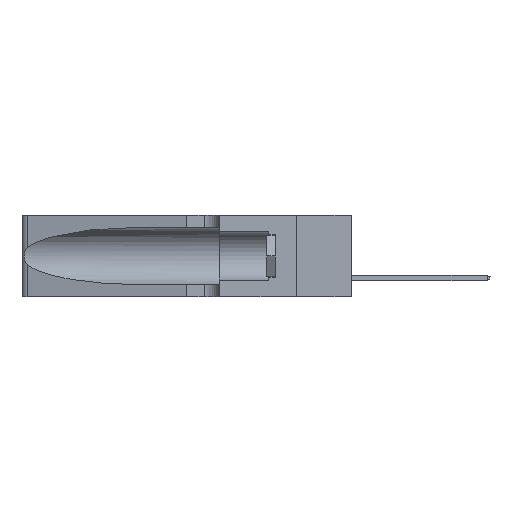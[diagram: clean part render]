
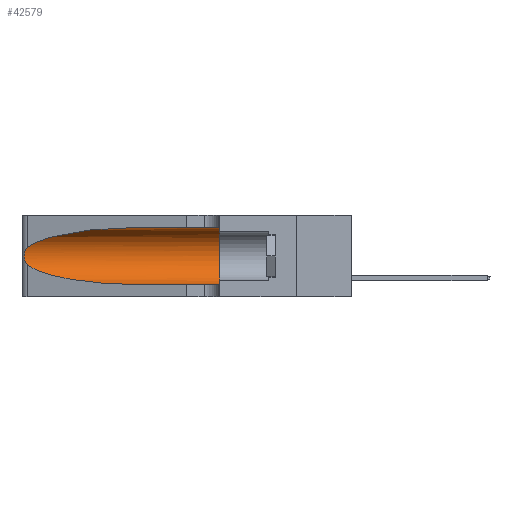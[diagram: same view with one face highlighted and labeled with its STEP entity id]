
A CAD part, left-side view. The second image highlights one B-rep face of the part: STEP entity #42579.
In plain terms, the highlighted cylindrical face has radius 3.308 mm (diameter 6.617 mm), a partial arc.
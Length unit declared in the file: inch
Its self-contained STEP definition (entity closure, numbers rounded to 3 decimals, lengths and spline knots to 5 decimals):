
#1730 = EDGE_LOOP ( 'NONE', ( #22844, #33410, #13693, #36216, #8523, #17052 ) ) ;
#2584 = DIRECTION ( 'NONE',  ( 0., -1., 0. ) ) ;
#3166 = CARTESIAN_POINT ( 'NONE',  ( 0.26075, 1.23896, 0.19203 ) ) ;
#6509 = VERTEX_POINT ( 'NONE', #18634 ) ;
#6924 = CARTESIAN_POINT ( 'NONE',  ( 0.1305, 1.61858, 0.05475 ) ) ;
#7042 = CARTESIAN_POINT ( 'NONE',  ( 0.25856, 1.23593, 0.16098 ) ) ;
#7304 = EDGE_CURVE ( 'NONE', #24124, #16155, #22294, .T. ) ;
#7346 = CARTESIAN_POINT ( 'NONE',  ( 0.25555, 1.22993, 0.14849 ) ) ;
#7727 = VERTEX_POINT ( 'NONE', #22287 ) ;
#8378 = DIRECTION ( 'NONE',  ( 0., 1., 0. ) ) ;
#8523 = ORIENTED_EDGE ( 'NONE', *, *, #11274, .F. ) ;
#9212 = CARTESIAN_POINT ( 'NONE',  ( 0.2373, 1.15595, 0.08982 ) ) ;
#10219 = CARTESIAN_POINT ( 'NONE',  ( 0.1305, 0.72297, 0.05475 ) ) ;
#10306 = DIRECTION ( 'NONE',  ( 0., -1., 0. ) ) ;
#11274 = EDGE_CURVE ( 'NONE', #6509, #7727, #36839, .T. ) ;
#12503 = CARTESIAN_POINT ( 'NONE',  ( 0.1305, 1.61858, 0.185 ) ) ;
#12618 = DIRECTION ( 'NONE',  ( 0., -1., 0. ) ) ;
#12716 = CARTESIAN_POINT ( 'NONE',  ( 0.1305, 0.72297, 0.05475 ) ) ;
#13086 = CARTESIAN_POINT ( 'NONE',  ( 0.25639, 1.23184, 0.21858 ) ) ;
#13378 = CARTESIAN_POINT ( 'NONE',  ( 0.25854, 1.2359, 0.20912 ) ) ;
#13693 = ORIENTED_EDGE ( 'NONE', *, *, #22281, .T. ) ;
#13729 = VERTEX_POINT ( 'NONE', #40265 ) ;
#13948 = EDGE_CURVE ( 'NONE', #16155, #13729, #35028, .T. ) ;
#14404 = VERTEX_POINT ( 'NONE', #10219 ) ;
#15712 = DIRECTION ( 'NONE',  ( 0., 0., -1. ) ) ;
#16155 = VERTEX_POINT ( 'NONE', #21185 ) ;
#16487 = CARTESIAN_POINT ( 'NONE',  ( 0.1305, 0.72297, 0.31525 ) ) ;
#16870 = CARTESIAN_POINT ( 'NONE',  ( 0.25787, 1.23484, 0.2124 ) ) ;
#17001 = CARTESIAN_POINT ( 'NONE',  ( 0.25789, 1.23486, 0.15765 ) ) ;
#17052 = ORIENTED_EDGE ( 'NONE', *, *, #36193, .F. ) ;
#18634 = CARTESIAN_POINT ( 'NONE',  ( 0.1305, 0.35, 0.31525 ) ) ;
#19123 = CARTESIAN_POINT ( 'NONE',  ( 0.25487, 1.22718, 0.22369 ) ) ;
#21185 = CARTESIAN_POINT ( 'NONE',  ( 0.25487, 1.22718, 0.22369 ) ) ;
#22281 = EDGE_CURVE ( 'NONE', #13729, #14404, #36347, .T. ) ;
#22287 = CARTESIAN_POINT ( 'NONE',  ( 0.1305, 0.35, 0.05475 ) ) ;
#22294 =( BOUNDED_CURVE ( )  B_SPLINE_CURVE ( 3, ( #16487, #30259, #33034, #23456 ),
 .UNSPECIFIED., .F., .T. ) 
 B_SPLINE_CURVE_WITH_KNOTS ( ( 4, 4 ),
 ( 1.5708, 2.84003 ),
 .UNSPECIFIED. ) 
 CURVE ( )  GEOMETRIC_REPRESENTATION_ITEM ( )  RATIONAL_B_SPLINE_CURVE ( ( 1., 0.87, 0.87, 1. ) ) 
 REPRESENTATION_ITEM ( '' )  );
#22844 = ORIENTED_EDGE ( 'NONE', *, *, #7304, .T. ) ;
#23456 = CARTESIAN_POINT ( 'NONE',  ( 0.25487, 1.22718, 0.22369 ) ) ;
#23699 = CARTESIAN_POINT ( 'NONE',  ( 0.26017, 1.23833, 0.17102 ) ) ;
#24088 = LINE ( 'NONE', #6924, #26220 ) ;
#24124 = VERTEX_POINT ( 'NONE', #25680 ) ;
#24942 = AXIS2_PLACEMENT_3D ( 'NONE', #12503, #2584, #15712 ) ;
#25680 = CARTESIAN_POINT ( 'NONE',  ( 0.1305, 0.72297, 0.31525 ) ) ;
#25812 = CARTESIAN_POINT ( 'NONE',  ( 0.25555, 1.22994, 0.2215 ) ) ;
#26220 = VECTOR ( 'NONE', #10306, 39.37008 ) ;
#28620 = DIRECTION ( 'NONE',  ( 0., 0., 1. ) ) ;
#28625 = CARTESIAN_POINT ( 'NONE',  ( 0.1305, 1.61858, 0.31525 ) ) ;
#29391 = VECTOR ( 'NONE', #12618, 39.37008 ) ;
#30259 = CARTESIAN_POINT ( 'NONE',  ( 0.18966, 0.96281, 0.31525 ) ) ;
#32503 = EDGE_CURVE ( 'NONE', #14404, #7727, #24088, .T. ) ;
#33034 = CARTESIAN_POINT ( 'NONE',  ( 0.2373, 1.15595, 0.28018 ) ) ;
#33410 = ORIENTED_EDGE ( 'NONE', *, *, #13948, .T. ) ;
#33814 = CARTESIAN_POINT ( 'NONE',  ( 0.25639, 1.23186, 0.15144 ) ) ;
#35028 = B_SPLINE_CURVE_WITH_KNOTS ( 'NONE', 3,
 ( #19123, #25812, #13086, #16870, #13378, #40082, #3166, #39946, #23699, #7042, #17001, #33814, #7346, #37144 ),
 .UNSPECIFIED., .F., .F.,
 ( 4, 2, 2, 2, 2, 2, 4 ),
 ( 0., 0.00027, 0.00053, 0.00107, 0.0016, 0.00187, 0.00214 ),
 .UNSPECIFIED. ) ;
#36193 = EDGE_CURVE ( 'NONE', #24124, #6509, #38196, .T. ) ;
#36207 = CARTESIAN_POINT ( 'NONE',  ( 0.18966, 0.96281, 0.05475 ) ) ;
#36216 = ORIENTED_EDGE ( 'NONE', *, *, #32503, .T. ) ;
#36347 =( BOUNDED_CURVE ( )  B_SPLINE_CURVE ( 3, ( #42505, #9212, #36207, #12716 ),
 .UNSPECIFIED., .F., .T. ) 
 B_SPLINE_CURVE_WITH_KNOTS ( ( 4, 4 ),
 ( 3.44316, 4.71239 ),
 .UNSPECIFIED. ) 
 CURVE ( )  GEOMETRIC_REPRESENTATION_ITEM ( )  RATIONAL_B_SPLINE_CURVE ( ( 1., 0.87, 0.87, 1. ) ) 
 REPRESENTATION_ITEM ( '' )  );
#36839 = CIRCLE ( 'NONE', #39809, 0.13025 ) ;
#37144 = CARTESIAN_POINT ( 'NONE',  ( 0.25487, 1.22718, 0.14631 ) ) ;
#38196 = LINE ( 'NONE', #28625, #29391 ) ;
#38612 = CARTESIAN_POINT ( 'NONE',  ( 0.1305, 0.35, 0.185 ) ) ;
#39809 = AXIS2_PLACEMENT_3D ( 'NONE', #38612, #8378, #28620 ) ;
#39946 = CARTESIAN_POINT ( 'NONE',  ( 0.26075, 1.23896, 0.178 ) ) ;
#40082 = CARTESIAN_POINT ( 'NONE',  ( 0.26018, 1.23835, 0.19895 ) ) ;
#40265 = CARTESIAN_POINT ( 'NONE',  ( 0.25487, 1.22718, 0.14631 ) ) ;
#41666 = FACE_OUTER_BOUND ( 'NONE', #1730, .T. ) ;
#42505 = CARTESIAN_POINT ( 'NONE',  ( 0.25487, 1.22718, 0.14631 ) ) ;
#42579 = ADVANCED_FACE ( 'NONE', ( #41666 ), #42700, .F. ) ;
#42700 = CYLINDRICAL_SURFACE ( 'NONE', #24942, 0.13025 ) ;
